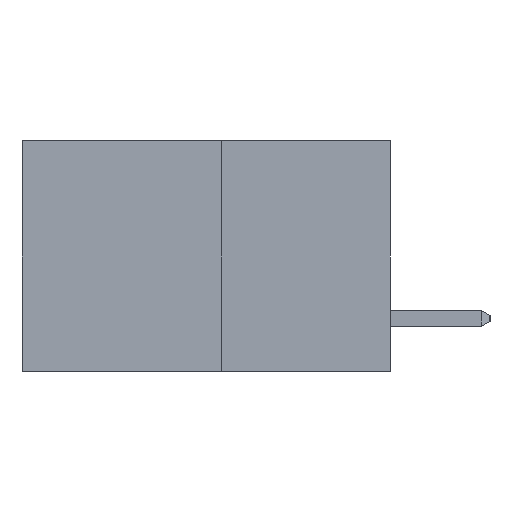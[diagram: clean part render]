
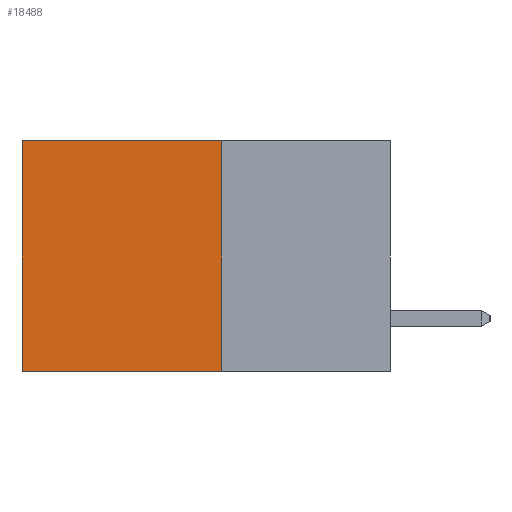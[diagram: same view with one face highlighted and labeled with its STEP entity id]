
A CAD part, left-side view. The second image highlights one B-rep face of the part: STEP entity #18488.
In plain terms, the highlighted planar face has unit normal (-1, 0, 0).
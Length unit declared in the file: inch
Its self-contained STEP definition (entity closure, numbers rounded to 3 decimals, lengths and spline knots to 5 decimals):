
#242 = LINE ( 'NONE', #24344, #11987 ) ;
#876 = CARTESIAN_POINT ( 'NONE',  ( 0.277, 0.27, -0.37 ) ) ;
#1249 = VERTEX_POINT ( 'NONE', #26155 ) ;
#2634 = DIRECTION ( 'NONE',  ( 1., 0., 0. ) ) ;
#4227 = VERTEX_POINT ( 'NONE', #876 ) ;
#4296 = VERTEX_POINT ( 'NONE', #6314 ) ;
#4646 = CARTESIAN_POINT ( 'NONE',  ( 0.277, 0.27, -0.37 ) ) ;
#4878 = FACE_OUTER_BOUND ( 'NONE', #18420, .T. ) ;
#5788 = DIRECTION ( 'NONE',  ( 0., 1., 0. ) ) ;
#5872 = CARTESIAN_POINT ( 'NONE',  ( 0.277, 0.27, 0. ) ) ;
#6314 = CARTESIAN_POINT ( 'NONE',  ( 0.277, 0.59, -0.37 ) ) ;
#7340 = DIRECTION ( 'NONE',  ( 0., 0., -1. ) ) ;
#7561 = VECTOR ( 'NONE', #8267, 39.37008 ) ;
#8267 = DIRECTION ( 'NONE',  ( 0., 1., 0. ) ) ;
#9790 = AXIS2_PLACEMENT_3D ( 'NONE', #27991, #2634, #18963 ) ;
#11987 = VECTOR ( 'NONE', #5788, 39.37008 ) ;
#12079 = VECTOR ( 'NONE', #7340, 39.37008 ) ;
#14477 = LINE ( 'NONE', #5872, #7561 ) ;
#18420 = EDGE_LOOP ( 'NONE', ( #25148, #22787, #19345, #27821 ) ) ;
#18488 = ADVANCED_FACE ( 'NONE', ( #4878 ), #21059, .F. ) ;
#18653 = DIRECTION ( 'NONE',  ( 0., 0., -1. ) ) ;
#18948 = CARTESIAN_POINT ( 'NONE',  ( 0.277, 0.59, -0.37 ) ) ;
#18963 = DIRECTION ( 'NONE',  ( 0., 0., -1. ) ) ;
#19345 = ORIENTED_EDGE ( 'NONE', *, *, #24498, .F. ) ;
#21059 = PLANE ( 'NONE',  #9790 ) ;
#21281 = CARTESIAN_POINT ( 'NONE',  ( 0.277, 0.27, 0. ) ) ;
#22504 = LINE ( 'NONE', #4646, #27098 ) ;
#22759 = EDGE_CURVE ( 'NONE', #1249, #4296, #24329, .T. ) ;
#22787 = ORIENTED_EDGE ( 'NONE', *, *, #28657, .F. ) ;
#24329 = LINE ( 'NONE', #18948, #12079 ) ;
#24344 = CARTESIAN_POINT ( 'NONE',  ( 0.277, 0.27, -0.37 ) ) ;
#24498 = EDGE_CURVE ( 'NONE', #28425, #4227, #22504, .T. ) ;
#25148 = ORIENTED_EDGE ( 'NONE', *, *, #22759, .T. ) ;
#26155 = CARTESIAN_POINT ( 'NONE',  ( 0.277, 0.59, 0. ) ) ;
#27098 = VECTOR ( 'NONE', #18653, 39.37008 ) ;
#27821 = ORIENTED_EDGE ( 'NONE', *, *, #29213, .T. ) ;
#27991 = CARTESIAN_POINT ( 'NONE',  ( 0.277, 0.27, -0.37 ) ) ;
#28425 = VERTEX_POINT ( 'NONE', #21281 ) ;
#28657 = EDGE_CURVE ( 'NONE', #4227, #4296, #242, .T. ) ;
#29213 = EDGE_CURVE ( 'NONE', #28425, #1249, #14477, .T. ) ;
